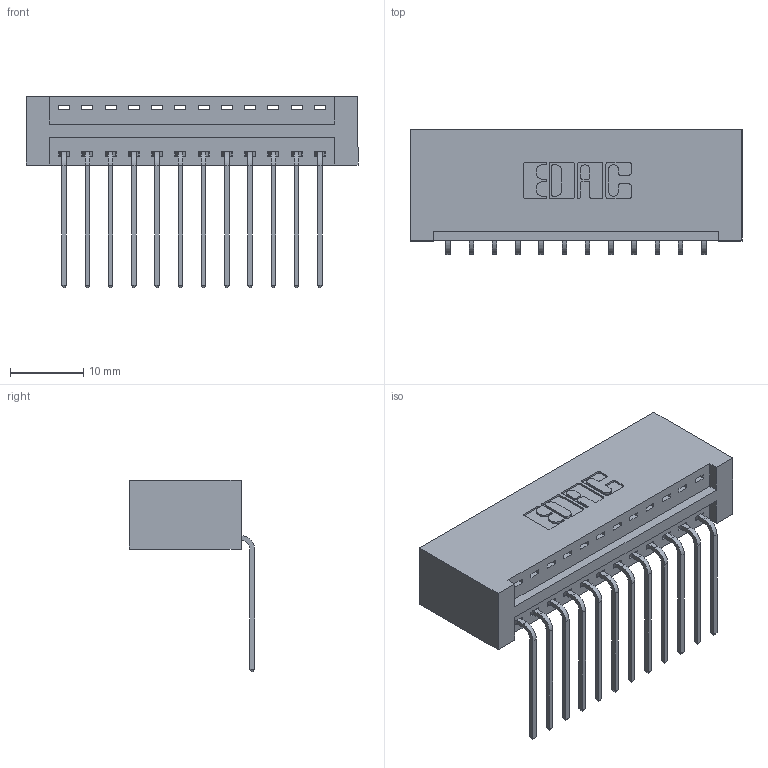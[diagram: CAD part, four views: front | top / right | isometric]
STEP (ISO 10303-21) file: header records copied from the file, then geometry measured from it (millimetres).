
FILE_DESCRIPTION (( 'STEP AP203' ), '1' );
FILE_NAME ('346-012-559-101.STEP', '2022-05-05T03:31:22', ( '' ), ( '' ), 'SwSTEP 2.0', 'SolidWorks 2020', '' );
FILE_SCHEMA (( 'CONFIG_CONTROL_DESIGN' ));
Length unit declared in the file: inch
Products named in the file (3): 346 Part_No Mounting Lugs; 346-012-559-101; 345-292-001_558 559 Tail - 1
Assembly tree (13 placements, depth 2):
  346-012-559-101
    346 Part_No Mounting Lugs
    345-292-001_558 559 Tail - 1  x12
Bounding box: 45.34 x 17.08 x 26.16 mm (x, y, z)
Volume: 4722.6 mm3; surface area: 5892.6 mm2
Topology: 13 solids, 13 shells, 834 faces, 2489 edges, 1642 vertices
Faces by surface type: plane 576, cylinder 258
Entity records: 11293 total; most frequent: CARTESIAN_POINT 1952, ORIENTED_EDGE 1898, DIRECTION 1753, EDGE_CURVE 949, VECTOR 777, LINE 777, VERTEX_POINT 630, AXIS2_PLACEMENT_3D 488
